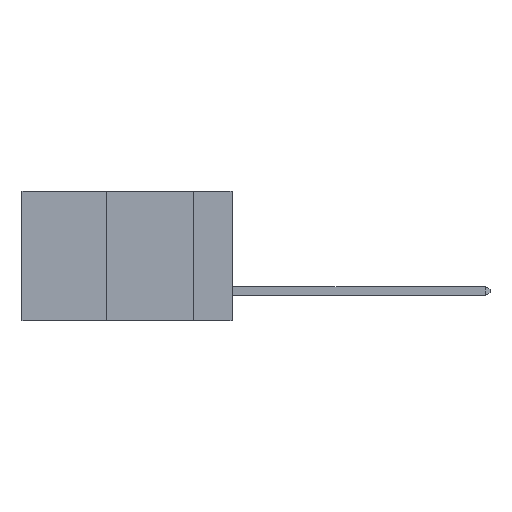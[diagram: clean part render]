
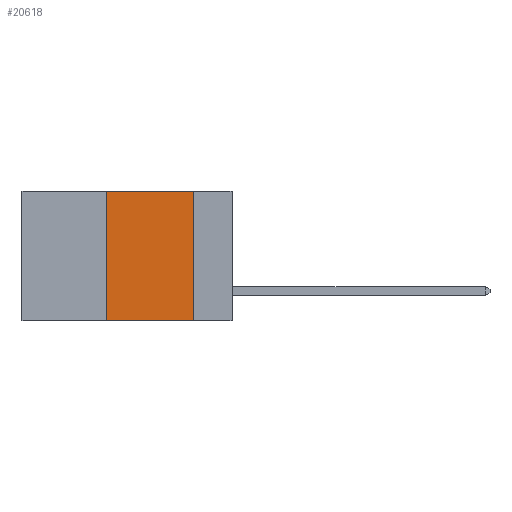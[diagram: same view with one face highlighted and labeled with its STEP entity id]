
A CAD part, left-side view. The second image highlights one B-rep face of the part: STEP entity #20618.
In plain terms, the highlighted planar face has unit normal (-1, 0, 0).
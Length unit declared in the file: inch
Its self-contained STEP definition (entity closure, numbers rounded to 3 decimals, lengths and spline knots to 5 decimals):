
#592 = CARTESIAN_POINT ( 'NONE',  ( 0., 0.11, -0.37 ) ) ;
#1018 = CARTESIAN_POINT ( 'NONE',  ( 0., 0.6, 0. ) ) ;
#1643 = EDGE_CURVE ( 'NONE', #7142, #2995, #15742, .T. ) ;
#2422 = LINE ( 'NONE', #24886, #23202 ) ;
#2725 = CARTESIAN_POINT ( 'NONE',  ( 0., 0.36, 0. ) ) ;
#2995 = VERTEX_POINT ( 'NONE', #12544 ) ;
#3109 = DIRECTION ( 'NONE',  ( 0., 0., -1. ) ) ;
#4857 = DIRECTION ( 'NONE',  ( 0., 0., 1. ) ) ;
#5654 = VECTOR ( 'NONE', #11117, 39.37008 ) ;
#6463 = CARTESIAN_POINT ( 'NONE',  ( 0., 0.36, -0.37 ) ) ;
#7142 = VERTEX_POINT ( 'NONE', #15551 ) ;
#8444 = ORIENTED_EDGE ( 'NONE', *, *, #12431, .F. ) ;
#8975 = LINE ( 'NONE', #2725, #18990 ) ;
#10648 = EDGE_LOOP ( 'NONE', ( #8444, #19106, #15067, #25477 ) ) ;
#11117 = DIRECTION ( 'NONE',  ( 0., -1., 0. ) ) ;
#11127 = DIRECTION ( 'NONE',  ( 0., 0., -1. ) ) ;
#11739 = VERTEX_POINT ( 'NONE', #592 ) ;
#12431 = EDGE_CURVE ( 'NONE', #2995, #11739, #2422, .T. ) ;
#12544 = CARTESIAN_POINT ( 'NONE',  ( 0., 0.11, 0. ) ) ;
#12615 = FACE_OUTER_BOUND ( 'NONE', #10648, .T. ) ;
#12941 = EDGE_CURVE ( 'NONE', #25520, #11739, #25823, .T. ) ;
#13268 = PLANE ( 'NONE',  #19408 ) ;
#15067 = ORIENTED_EDGE ( 'NONE', *, *, #16981, .F. ) ;
#15275 = DIRECTION ( 'NONE',  ( 1., 0., 0. ) ) ;
#15551 = CARTESIAN_POINT ( 'NONE',  ( 0., 0.36, 0. ) ) ;
#15742 = LINE ( 'NONE', #19781, #5654 ) ;
#16657 = CARTESIAN_POINT ( 'NONE',  ( 0., 0.6, -0.37 ) ) ;
#16981 = EDGE_CURVE ( 'NONE', #25520, #7142, #8975, .T. ) ;
#18990 = VECTOR ( 'NONE', #4857, 39.37008 ) ;
#19106 = ORIENTED_EDGE ( 'NONE', *, *, #1643, .F. ) ;
#19408 = AXIS2_PLACEMENT_3D ( 'NONE', #1018, #15275, #3109 ) ;
#19781 = CARTESIAN_POINT ( 'NONE',  ( 0., 0.6, 0. ) ) ;
#20618 = ADVANCED_FACE ( 'NONE', ( #12615 ), #13268, .F. ) ;
#20686 = VECTOR ( 'NONE', #24519, 39.37008 ) ;
#23202 = VECTOR ( 'NONE', #11127, 39.37008 ) ;
#24519 = DIRECTION ( 'NONE',  ( 0., -1., 0. ) ) ;
#24886 = CARTESIAN_POINT ( 'NONE',  ( 0., 0.11, 0. ) ) ;
#25477 = ORIENTED_EDGE ( 'NONE', *, *, #12941, .T. ) ;
#25520 = VERTEX_POINT ( 'NONE', #6463 ) ;
#25823 = LINE ( 'NONE', #16657, #20686 ) ;
